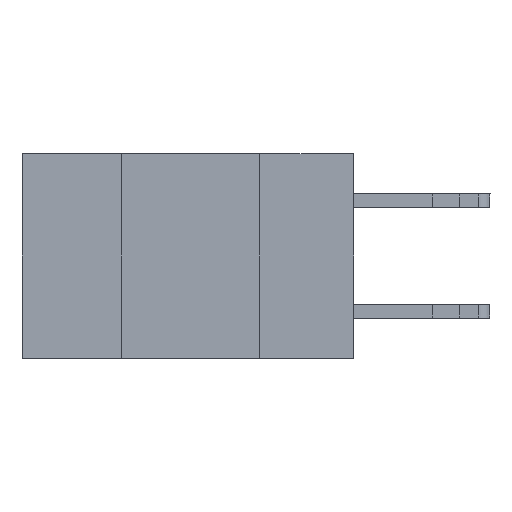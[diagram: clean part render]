
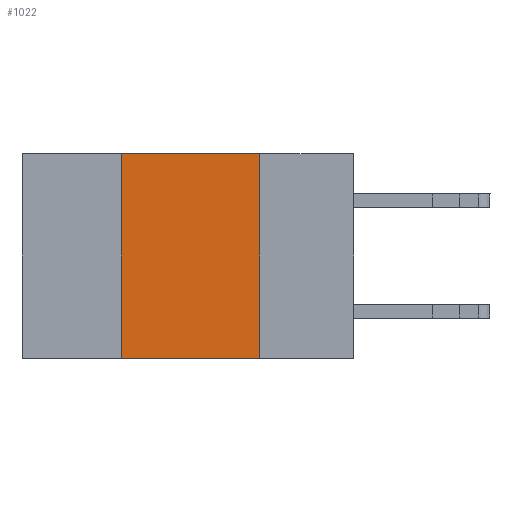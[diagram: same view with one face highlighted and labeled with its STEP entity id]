
A CAD part, left-side view. The second image highlights one B-rep face of the part: STEP entity #1022.
In plain terms, the highlighted planar face has unit normal (-1, 0, 0).
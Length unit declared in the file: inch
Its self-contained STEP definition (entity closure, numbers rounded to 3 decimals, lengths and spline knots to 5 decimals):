
#330 = CARTESIAN_POINT ( 'NONE',  ( 0., 0.6, 0. ) ) ;
#804 = LINE ( 'NONE', #4126, #18414 ) ;
#1022 = ADVANCED_FACE ( 'NONE', ( #1721 ), #19153, .F. ) ;
#1172 = ORIENTED_EDGE ( 'NONE', *, *, #21909, .F. ) ;
#1494 = CARTESIAN_POINT ( 'NONE',  ( 0., 0.6, 0. ) ) ;
#1721 = FACE_OUTER_BOUND ( 'NONE', #12311, .T. ) ;
#2494 = EDGE_CURVE ( 'NONE', #19146, #20488, #13644, .T. ) ;
#4086 = VECTOR ( 'NONE', #12458, 39.37008 ) ;
#4126 = CARTESIAN_POINT ( 'NONE',  ( 0., 0.6, -0.37 ) ) ;
#5251 = CARTESIAN_POINT ( 'NONE',  ( 0., 0.17, 0. ) ) ;
#5372 = LINE ( 'NONE', #5251, #4086 ) ;
#6606 = AXIS2_PLACEMENT_3D ( 'NONE', #330, #9080, #10784 ) ;
#6622 = ORIENTED_EDGE ( 'NONE', *, *, #8792, .F. ) ;
#7589 = CARTESIAN_POINT ( 'NONE',  ( 0., 0.42, -0.37 ) ) ;
#8792 = EDGE_CURVE ( 'NONE', #21650, #19146, #22579, .T. ) ;
#9079 = DIRECTION ( 'NONE',  ( 0., -1., 0. ) ) ;
#9080 = DIRECTION ( 'NONE',  ( 1., 0., 0. ) ) ;
#9271 = VECTOR ( 'NONE', #20735, 39.37008 ) ;
#9423 = CARTESIAN_POINT ( 'NONE',  ( 0., 0.17, -0.37 ) ) ;
#10049 = VERTEX_POINT ( 'NONE', #9423 ) ;
#10784 = DIRECTION ( 'NONE',  ( 0., 0., -1. ) ) ;
#11690 = CARTESIAN_POINT ( 'NONE',  ( 0., 0.42, 0. ) ) ;
#11859 = DIRECTION ( 'NONE',  ( 0., 0., 1. ) ) ;
#12311 = EDGE_LOOP ( 'NONE', ( #1172, #22582, #6622, #20557 ) ) ;
#12458 = DIRECTION ( 'NONE',  ( 0., 0., -1. ) ) ;
#13644 = LINE ( 'NONE', #1494, #9271 ) ;
#16427 = VECTOR ( 'NONE', #11859, 39.37008 ) ;
#18414 = VECTOR ( 'NONE', #9079, 39.37008 ) ;
#19146 = VERTEX_POINT ( 'NONE', #11690 ) ;
#19153 = PLANE ( 'NONE',  #6606 ) ;
#19423 = CARTESIAN_POINT ( 'NONE',  ( 0., 0.17, 0. ) ) ;
#20488 = VERTEX_POINT ( 'NONE', #19423 ) ;
#20557 = ORIENTED_EDGE ( 'NONE', *, *, #22575, .T. ) ;
#20735 = DIRECTION ( 'NONE',  ( 0., -1., 0. ) ) ;
#20998 = CARTESIAN_POINT ( 'NONE',  ( 0., 0.42, 0. ) ) ;
#21650 = VERTEX_POINT ( 'NONE', #7589 ) ;
#21909 = EDGE_CURVE ( 'NONE', #20488, #10049, #5372, .T. ) ;
#22575 = EDGE_CURVE ( 'NONE', #21650, #10049, #804, .T. ) ;
#22579 = LINE ( 'NONE', #20998, #16427 ) ;
#22582 = ORIENTED_EDGE ( 'NONE', *, *, #2494, .F. ) ;
